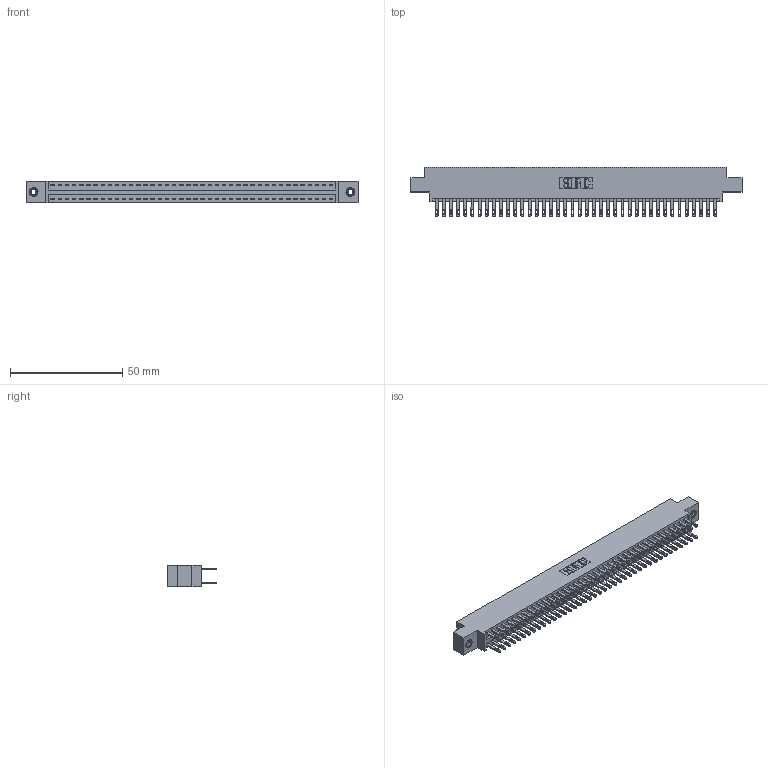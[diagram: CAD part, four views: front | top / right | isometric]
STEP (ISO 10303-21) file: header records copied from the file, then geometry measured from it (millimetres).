
FILE_DESCRIPTION (( 'STEP AP203' ), '1' );
FILE_NAME ('896-080-500-808.STEP', '2021-07-28T02:07:50', ( '' ), ( '' ), 'SwSTEP 2.0', 'SolidWorks 2020', '' );
FILE_SCHEMA (( 'CONFIG_CONTROL_DESIGN' ));
Length unit declared in the file: inch
Products named in the file (4): 345-250-001_345-250-003-102; 846 Part_0.170 Offset - 0.156 Dia-TI; 896-080-500-808; 345-292-001_345-293-100
Assembly tree (83 placements, depth 2):
  896-080-500-808
    846 Part_0.170 Offset - 0.156 Dia-TI
    345-292-001_345-293-100  x80
    345-250-001_345-250-003-102  x2
Bounding box: 147.57 x 21.84 x 9.4 mm (x, y, z)
Volume: 14458.1 mm3; surface area: 20879.2 mm2
Topology: 83 solids, 83 shells, 4026 faces, 12237 edges, 8150 vertices
Faces by surface type: plane 2432, cylinder 1578, cone 12, torus 4
Entity records: 27622 total; most frequent: CARTESIAN_POINT 4539, ORIENTED_EDGE 4466, DIRECTION 4079, EDGE_CURVE 2233, LINE 1917, VECTOR 1917, VERTEX_POINT 1484, AXIS2_PLACEMENT_3D 1081
